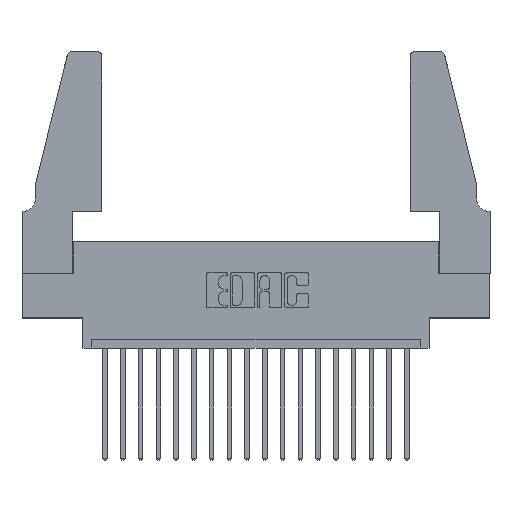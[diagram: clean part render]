
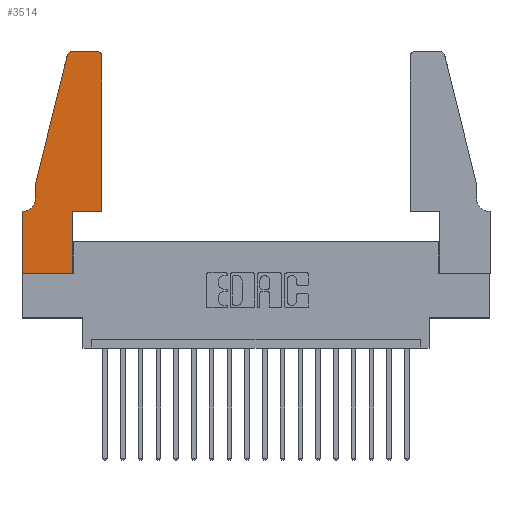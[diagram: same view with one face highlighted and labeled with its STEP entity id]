
A CAD part, top view. The second image highlights one B-rep face of the part: STEP entity #3514.
In plain terms, the highlighted planar face has unit normal (0, 0, 1).
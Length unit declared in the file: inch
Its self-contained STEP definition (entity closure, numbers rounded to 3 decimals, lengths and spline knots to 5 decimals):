
#135 = VECTOR ( 'NONE', #192, 39.37008 ) ;
#192 = DIRECTION ( 'NONE',  ( -0.239, -0.971, 0. ) ) ;
#233 = VECTOR ( 'NONE', #5444, 39.37008 ) ;
#304 = ORIENTED_EDGE ( 'NONE', *, *, #654, .T. ) ;
#654 = EDGE_CURVE ( 'NONE', #4525, #5848, #9133, .T. ) ;
#867 = CARTESIAN_POINT ( 'NONE',  ( 0.4205, 1.25, 0.37 ) ) ;
#1051 = VECTOR ( 'NONE', #8833, 39.37008 ) ;
#1075 = LINE ( 'NONE', #12423, #14166 ) ;
#1199 = ORIENTED_EDGE ( 'NONE', *, *, #17950, .T. ) ;
#1524 = CARTESIAN_POINT ( 'NONE',  ( 0., 0.35, 0.37 ) ) ;
#1776 = CIRCLE ( 'NONE', #3085, 0.07 ) ;
#2034 = ORIENTED_EDGE ( 'NONE', *, *, #13998, .T. ) ;
#2287 = DIRECTION ( 'NONE',  ( 0., 1., 0. ) ) ;
#3085 = AXIS2_PLACEMENT_3D ( 'NONE', #12069, #10687, #14801 ) ;
#3514 = ADVANCED_FACE ( 'NONE', ( #13310 ), #15551, .T. ) ;
#3779 = DIRECTION ( 'NONE',  ( 1., 0., 0. ) ) ;
#3836 = CARTESIAN_POINT ( 'NONE',  ( 0.284, 1.25, 0.37 ) ) ;
#3968 = VERTEX_POINT ( 'NONE', #5697 ) ;
#4121 = VERTEX_POINT ( 'NONE', #15593 ) ;
#4159 = CARTESIAN_POINT ( 'NONE',  ( 0.2865, 0., 0.37 ) ) ;
#4326 = DIRECTION ( 'NONE',  ( 0., 1., 0. ) ) ;
#4525 = VERTEX_POINT ( 'NONE', #3836 ) ;
#4688 = CARTESIAN_POINT ( 'NONE',  ( 0.0755, 0.5, 0.37 ) ) ;
#4700 = CARTESIAN_POINT ( 'NONE',  ( 0.0755, 0.35, 0.37 ) ) ;
#4953 = LINE ( 'NONE', #9024, #1051 ) ;
#5062 = EDGE_CURVE ( 'NONE', #16123, #18219, #6355, .T. ) ;
#5065 = DIRECTION ( 'NONE',  ( 0., 0., 1. ) ) ;
#5106 = VERTEX_POINT ( 'NONE', #8702 ) ;
#5276 = LINE ( 'NONE', #4700, #9190 ) ;
#5333 = ORIENTED_EDGE ( 'NONE', *, *, #15902, .T. ) ;
#5444 = DIRECTION ( 'NONE',  ( -1., 0., 0. ) ) ;
#5697 = CARTESIAN_POINT ( 'NONE',  ( 0.0755, 0.5, 0.37 ) ) ;
#5754 = LINE ( 'NONE', #7386, #13553 ) ;
#5848 = VERTEX_POINT ( 'NONE', #13760 ) ;
#6190 = VERTEX_POINT ( 'NONE', #16804 ) ;
#6245 = AXIS2_PLACEMENT_3D ( 'NONE', #7962, #15496, #9507 ) ;
#6355 = LINE ( 'NONE', #18407, #10038 ) ;
#6519 = CARTESIAN_POINT ( 'NONE',  ( 0.4505, 0.35, 0.37 ) ) ;
#6848 = CARTESIAN_POINT ( 'NONE',  ( 0.2605, 1.25, 0.37 ) ) ;
#7197 = EDGE_CURVE ( 'NONE', #18219, #6190, #11320, .T. ) ;
#7286 = LINE ( 'NONE', #8749, #8901 ) ;
#7319 = ORIENTED_EDGE ( 'NONE', *, *, #9659, .T. ) ;
#7386 = CARTESIAN_POINT ( 'NONE',  ( 0.0755, 0.5, 0.37 ) ) ;
#7454 = VERTEX_POINT ( 'NONE', #1524 ) ;
#7596 = CIRCLE ( 'NONE', #6245, 0.03 ) ;
#7962 = CARTESIAN_POINT ( 'NONE',  ( 0.4205, 1.22, 0.37 ) ) ;
#8139 = CARTESIAN_POINT ( 'NONE',  ( 0.284, 1.22, 0.37 ) ) ;
#8308 = LINE ( 'NONE', #6848, #233 ) ;
#8415 = VERTEX_POINT ( 'NONE', #867 ) ;
#8443 = LINE ( 'NONE', #4688, #135 ) ;
#8478 = AXIS2_PLACEMENT_3D ( 'NONE', #13925, #5065, #9566 ) ;
#8493 = CARTESIAN_POINT ( 'NONE',  ( 0.0755, 0.42, 0.37 ) ) ;
#8587 = VERTEX_POINT ( 'NONE', #8493 ) ;
#8702 = CARTESIAN_POINT ( 'NONE',  ( 0.0055, 0.35, 0.37 ) ) ;
#8749 = CARTESIAN_POINT ( 'NONE',  ( 0., 0., 0.37 ) ) ;
#8833 = DIRECTION ( 'NONE',  ( 1., 0., 0. ) ) ;
#8901 = VECTOR ( 'NONE', #13147, 39.37008 ) ;
#9024 = CARTESIAN_POINT ( 'NONE',  ( 0.4505, 0.35, 0.37 ) ) ;
#9050 = ORIENTED_EDGE ( 'NONE', *, *, #14487, .T. ) ;
#9133 = CIRCLE ( 'NONE', #15246, 0.03 ) ;
#9190 = VECTOR ( 'NONE', #11996, 39.37008 ) ;
#9507 = DIRECTION ( 'NONE',  ( 1., 0., 0. ) ) ;
#9566 = DIRECTION ( 'NONE',  ( 1., 0., 0. ) ) ;
#9635 = ORIENTED_EDGE ( 'NONE', *, *, #16245, .T. ) ;
#9659 = EDGE_CURVE ( 'NONE', #7454, #16123, #7286, .T. ) ;
#9975 = EDGE_CURVE ( 'NONE', #5848, #3968, #8443, .T. ) ;
#10038 = VECTOR ( 'NONE', #3779, 39.37008 ) ;
#10687 = DIRECTION ( 'NONE',  ( 0., 0., -1. ) ) ;
#11118 = DIRECTION ( 'NONE',  ( 1., 0., 0. ) ) ;
#11320 = LINE ( 'NONE', #13112, #12476 ) ;
#11734 = ORIENTED_EDGE ( 'NONE', *, *, #5062, .T. ) ;
#11921 = VERTEX_POINT ( 'NONE', #6519 ) ;
#11996 = DIRECTION ( 'NONE',  ( -1., 0., 0. ) ) ;
#12069 = CARTESIAN_POINT ( 'NONE',  ( 0.0055, 0.42, 0.37 ) ) ;
#12221 = CARTESIAN_POINT ( 'NONE',  ( 0., 0., 0.37 ) ) ;
#12423 = CARTESIAN_POINT ( 'NONE',  ( 0.4505, 0.35, 0.37 ) ) ;
#12476 = VECTOR ( 'NONE', #4326, 39.37008 ) ;
#12668 = DIRECTION ( 'NONE',  ( 0., 0., 1. ) ) ;
#13112 = CARTESIAN_POINT ( 'NONE',  ( 0.2865, 0.35, 0.37 ) ) ;
#13147 = DIRECTION ( 'NONE',  ( 0., -1., 0. ) ) ;
#13310 = FACE_OUTER_BOUND ( 'NONE', #14243, .T. ) ;
#13553 = VECTOR ( 'NONE', #15942, 39.37008 ) ;
#13760 = CARTESIAN_POINT ( 'NONE',  ( 0.25487, 1.22718, 0.37 ) ) ;
#13925 = CARTESIAN_POINT ( 'NONE',  ( 0., 0.35, 0.37 ) ) ;
#13998 = EDGE_CURVE ( 'NONE', #4121, #8415, #7596, .T. ) ;
#14166 = VECTOR ( 'NONE', #2287, 39.37008 ) ;
#14243 = EDGE_LOOP ( 'NONE', ( #5333, #304, #16211, #9635, #1199, #9050, #7319, #11734, #16771, #16639, #16263, #2034 ) ) ;
#14487 = EDGE_CURVE ( 'NONE', #5106, #7454, #5276, .T. ) ;
#14801 = DIRECTION ( 'NONE',  ( -1., 0., 0. ) ) ;
#15246 = AXIS2_PLACEMENT_3D ( 'NONE', #8139, #12668, #11118 ) ;
#15496 = DIRECTION ( 'NONE',  ( 0., 0., 1. ) ) ;
#15551 = PLANE ( 'NONE',  #8478 ) ;
#15593 = CARTESIAN_POINT ( 'NONE',  ( 0.4505, 1.22, 0.37 ) ) ;
#15902 = EDGE_CURVE ( 'NONE', #8415, #4525, #8308, .T. ) ;
#15942 = DIRECTION ( 'NONE',  ( 0., -1., 0. ) ) ;
#16123 = VERTEX_POINT ( 'NONE', #12221 ) ;
#16211 = ORIENTED_EDGE ( 'NONE', *, *, #9975, .T. ) ;
#16245 = EDGE_CURVE ( 'NONE', #3968, #8587, #5754, .T. ) ;
#16263 = ORIENTED_EDGE ( 'NONE', *, *, #18112, .T. ) ;
#16639 = ORIENTED_EDGE ( 'NONE', *, *, #18300, .T. ) ;
#16771 = ORIENTED_EDGE ( 'NONE', *, *, #7197, .T. ) ;
#16804 = CARTESIAN_POINT ( 'NONE',  ( 0.2865, 0.35, 0.37 ) ) ;
#17950 = EDGE_CURVE ( 'NONE', #8587, #5106, #1776, .T. ) ;
#18112 = EDGE_CURVE ( 'NONE', #11921, #4121, #1075, .T. ) ;
#18219 = VERTEX_POINT ( 'NONE', #4159 ) ;
#18300 = EDGE_CURVE ( 'NONE', #6190, #11921, #4953, .T. ) ;
#18407 = CARTESIAN_POINT ( 'NONE',  ( 0., 0., 0.37 ) ) ;
